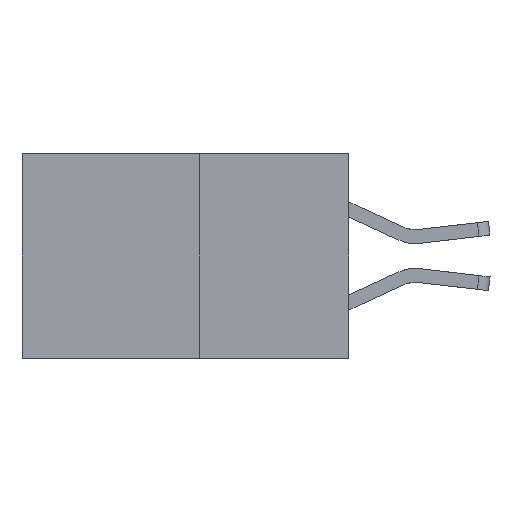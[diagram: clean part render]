
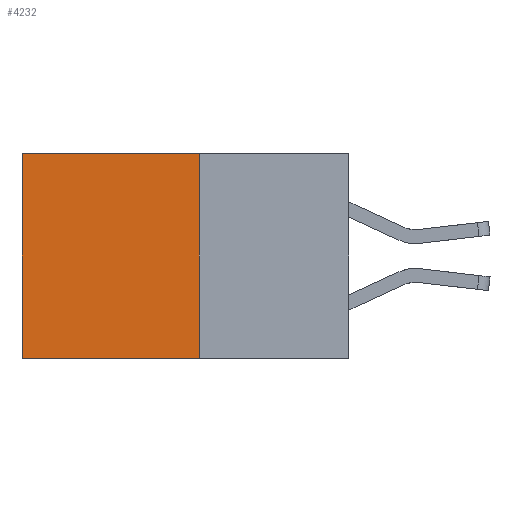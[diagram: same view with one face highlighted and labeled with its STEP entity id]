
A CAD part, left-side view. The second image highlights one B-rep face of the part: STEP entity #4232.
In plain terms, the highlighted planar face has unit normal (-1, 0, 0).
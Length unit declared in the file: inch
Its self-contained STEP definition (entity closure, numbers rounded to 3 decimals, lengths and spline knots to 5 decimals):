
#190 = CARTESIAN_POINT ( 'NONE',  ( 0.277, 0.59, 0. ) ) ;
#633 = LINE ( 'NONE', #8111, #5255 ) ;
#3179 = CARTESIAN_POINT ( 'NONE',  ( 0.277, 0.59, -0.37 ) ) ;
#3440 = VERTEX_POINT ( 'NONE', #8174 ) ;
#3702 = LINE ( 'NONE', #6121, #7865 ) ;
#3827 = DIRECTION ( 'NONE',  ( 1., 0., 0. ) ) ;
#4232 = ADVANCED_FACE ( 'NONE', ( #10706 ), #7124, .F. ) ;
#4404 = EDGE_CURVE ( 'NONE', #5939, #9908, #9469, .T. ) ;
#4720 = EDGE_CURVE ( 'NONE', #5755, #9908, #7638, .T. ) ;
#4794 = DIRECTION ( 'NONE',  ( 0., 0., -1. ) ) ;
#5255 = VECTOR ( 'NONE', #4794, 39.37008 ) ;
#5283 = EDGE_LOOP ( 'NONE', ( #8202, #8119, #6487, #5906 ) ) ;
#5306 = DIRECTION ( 'NONE',  ( 0., 1., 0. ) ) ;
#5424 = VECTOR ( 'NONE', #6699, 39.37008 ) ;
#5755 = VERTEX_POINT ( 'NONE', #6648 ) ;
#5846 = CARTESIAN_POINT ( 'NONE',  ( 0.277, 0.27, -0.37 ) ) ;
#5906 = ORIENTED_EDGE ( 'NONE', *, *, #10414, .T. ) ;
#5939 = VERTEX_POINT ( 'NONE', #190 ) ;
#6121 = CARTESIAN_POINT ( 'NONE',  ( 0.277, 0.27, 0. ) ) ;
#6487 = ORIENTED_EDGE ( 'NONE', *, *, #10793, .F. ) ;
#6543 = CARTESIAN_POINT ( 'NONE',  ( 0.277, 0.59, -0.37 ) ) ;
#6648 = CARTESIAN_POINT ( 'NONE',  ( 0.277, 0.27, -0.37 ) ) ;
#6699 = DIRECTION ( 'NONE',  ( 0., 1., 0. ) ) ;
#7124 = PLANE ( 'NONE',  #8808 ) ;
#7638 = LINE ( 'NONE', #5846, #5424 ) ;
#7865 = VECTOR ( 'NONE', #5306, 39.37008 ) ;
#8111 = CARTESIAN_POINT ( 'NONE',  ( 0.277, 0.27, -0.37 ) ) ;
#8119 = ORIENTED_EDGE ( 'NONE', *, *, #4720, .F. ) ;
#8174 = CARTESIAN_POINT ( 'NONE',  ( 0.277, 0.27, 0. ) ) ;
#8202 = ORIENTED_EDGE ( 'NONE', *, *, #4404, .T. ) ;
#8808 = AXIS2_PLACEMENT_3D ( 'NONE', #8834, #3827, #9645 ) ;
#8834 = CARTESIAN_POINT ( 'NONE',  ( 0.277, 0.27, -0.37 ) ) ;
#9011 = DIRECTION ( 'NONE',  ( 0., 0., -1. ) ) ;
#9469 = LINE ( 'NONE', #3179, #10446 ) ;
#9645 = DIRECTION ( 'NONE',  ( 0., 0., -1. ) ) ;
#9908 = VERTEX_POINT ( 'NONE', #6543 ) ;
#10414 = EDGE_CURVE ( 'NONE', #3440, #5939, #3702, .T. ) ;
#10446 = VECTOR ( 'NONE', #9011, 39.37008 ) ;
#10706 = FACE_OUTER_BOUND ( 'NONE', #5283, .T. ) ;
#10793 = EDGE_CURVE ( 'NONE', #3440, #5755, #633, .T. ) ;
